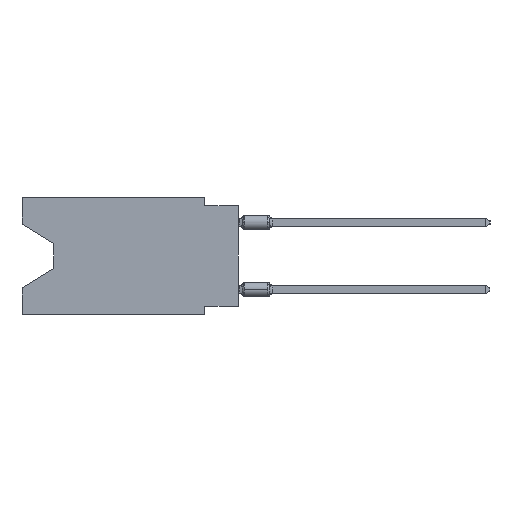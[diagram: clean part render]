
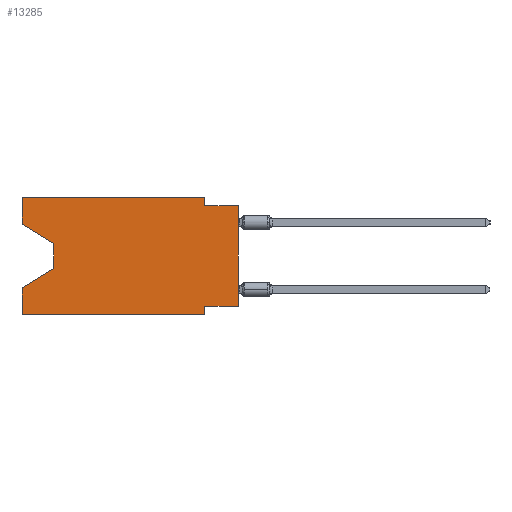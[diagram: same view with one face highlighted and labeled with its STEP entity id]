
A CAD part, left-side view. The second image highlights one B-rep face of the part: STEP entity #13285.
In plain terms, the highlighted planar face has unit normal (-1, 0, 0).
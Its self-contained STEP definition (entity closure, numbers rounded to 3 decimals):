
#343 = ORIENTED_EDGE ( 'NONE', *, *, #43292, .F. ) ;
#811 = CARTESIAN_POINT ( 'NONE',  ( 0., 16.383, 0. ) ) ;
#838 = LINE ( 'NONE', #42924, #15543 ) ;
#1033 = VERTEX_POINT ( 'NONE', #21829 ) ;
#1484 = EDGE_CURVE ( 'NONE', #16637, #2525, #44673, .T. ) ;
#1725 = LINE ( 'NONE', #29605, #27067 ) ;
#2525 = VERTEX_POINT ( 'NONE', #28909 ) ;
#2679 = CARTESIAN_POINT ( 'NONE',  ( 0., 16.383, -2.038 ) ) ;
#2691 = ORIENTED_EDGE ( 'NONE', *, *, #10028, .F. ) ;
#3459 = CARTESIAN_POINT ( 'NONE',  ( 0., 13.97, -5.385 ) ) ;
#3548 = EDGE_CURVE ( 'NONE', #30534, #17554, #838, .T. ) ;
#3558 = LINE ( 'NONE', #811, #14424 ) ;
#4808 = LINE ( 'NONE', #44132, #27550 ) ;
#5252 = CARTESIAN_POINT ( 'NONE',  ( 0., 2.54, -8.89 ) ) ;
#5733 = VECTOR ( 'NONE', #19193, 1000. ) ;
#7561 = DIRECTION ( 'NONE',  ( 0., 0., -1. ) ) ;
#7698 = ORIENTED_EDGE ( 'NONE', *, *, #27133, .F. ) ;
#7884 = CARTESIAN_POINT ( 'NONE',  ( 0., 0., -8.255 ) ) ;
#8462 = ORIENTED_EDGE ( 'NONE', *, *, #21504, .T. ) ;
#8587 = VERTEX_POINT ( 'NONE', #20730 ) ;
#9474 = DIRECTION ( 'NONE',  ( 0., -1., 0. ) ) ;
#9531 = CARTESIAN_POINT ( 'NONE',  ( 0., 2.54, -8.255 ) ) ;
#9591 = DIRECTION ( 'NONE',  ( 0., 0., 1. ) ) ;
#10028 = EDGE_CURVE ( 'NONE', #37496, #35633, #38396, .T. ) ;
#10310 = LINE ( 'NONE', #3459, #37599 ) ;
#10684 = ORIENTED_EDGE ( 'NONE', *, *, #33413, .T. ) ;
#11477 = CARTESIAN_POINT ( 'NONE',  ( 0., 13.97, -3.505 ) ) ;
#11752 = ORIENTED_EDGE ( 'NONE', *, *, #21544, .F. ) ;
#12558 = DIRECTION ( 'NONE',  ( 0., 0., 1. ) ) ;
#12906 = LINE ( 'NONE', #26847, #31722 ) ;
#13285 = ADVANCED_FACE ( 'NONE', ( #38209 ), #27908, .F. ) ;
#13310 = DIRECTION ( 'NONE',  ( 0., 0., -1. ) ) ;
#13400 = EDGE_CURVE ( 'NONE', #35983, #1033, #30785, .T. ) ;
#13512 = VECTOR ( 'NONE', #13310, 1000. ) ;
#13715 = EDGE_CURVE ( 'NONE', #35983, #8587, #1725, .T. ) ;
#13785 = VERTEX_POINT ( 'NONE', #16126 ) ;
#14193 = CARTESIAN_POINT ( 'NONE',  ( 0., 16.383, 0. ) ) ;
#14424 = VECTOR ( 'NONE', #21159, 1000. ) ;
#15543 = VECTOR ( 'NONE', #32831, 1000. ) ;
#15693 = VERTEX_POINT ( 'NONE', #9531 ) ;
#16126 = CARTESIAN_POINT ( 'NONE',  ( 0., 0., -8.255 ) ) ;
#16188 = VECTOR ( 'NONE', #39657, 1000. ) ;
#16637 = VERTEX_POINT ( 'NONE', #11477 ) ;
#17009 = ORIENTED_EDGE ( 'NONE', *, *, #3548, .F. ) ;
#17554 = VERTEX_POINT ( 'NONE', #37982 ) ;
#17857 = CARTESIAN_POINT ( 'NONE',  ( 0., 0., -0.635 ) ) ;
#19193 = DIRECTION ( 'NONE',  ( 0., 0., -1. ) ) ;
#19776 = CARTESIAN_POINT ( 'NONE',  ( 0., 16.383, 0. ) ) ;
#20458 = VERTEX_POINT ( 'NONE', #17857 ) ;
#20730 = CARTESIAN_POINT ( 'NONE',  ( 0., 2.54, -8.89 ) ) ;
#20774 = EDGE_LOOP ( 'NONE', ( #22227, #24663, #10684, #29657, #33717, #11752, #7698, #8462, #44574, #17009, #343, #2691 ) ) ;
#21159 = DIRECTION ( 'NONE',  ( 0., -1., 0. ) ) ;
#21504 = EDGE_CURVE ( 'NONE', #13785, #20458, #25608, .T. ) ;
#21544 = EDGE_CURVE ( 'NONE', #15693, #8587, #36564, .T. ) ;
#21829 = CARTESIAN_POINT ( 'NONE',  ( 0., 16.383, -6.852 ) ) ;
#22227 = ORIENTED_EDGE ( 'NONE', *, *, #43879, .T. ) ;
#24663 = ORIENTED_EDGE ( 'NONE', *, *, #1484, .T. ) ;
#25608 = LINE ( 'NONE', #43911, #44466 ) ;
#26198 = VECTOR ( 'NONE', #9591, 1000. ) ;
#26293 = AXIS2_PLACEMENT_3D ( 'NONE', #14193, #27689, #7561 ) ;
#26356 = CARTESIAN_POINT ( 'NONE',  ( 0., 16.383, -8.89 ) ) ;
#26721 = DIRECTION ( 'NONE',  ( 0., -0.855, -0.519 ) ) ;
#26847 = CARTESIAN_POINT ( 'NONE',  ( 0., 0., -0.635 ) ) ;
#26969 = CARTESIAN_POINT ( 'NONE',  ( 0., 16.383, 0. ) ) ;
#27067 = VECTOR ( 'NONE', #36921, 1000. ) ;
#27133 = EDGE_CURVE ( 'NONE', #13785, #15693, #36216, .T. ) ;
#27550 = VECTOR ( 'NONE', #26721, 1000. ) ;
#27689 = DIRECTION ( 'NONE',  ( 1., 0., 0. ) ) ;
#27789 = VECTOR ( 'NONE', #41088, 1000. ) ;
#27908 = PLANE ( 'NONE',  #26293 ) ;
#28909 = CARTESIAN_POINT ( 'NONE',  ( 0., 13.97, -5.385 ) ) ;
#29605 = CARTESIAN_POINT ( 'NONE',  ( 0., 16.383, -8.89 ) ) ;
#29657 = ORIENTED_EDGE ( 'NONE', *, *, #13400, .F. ) ;
#30534 = VERTEX_POINT ( 'NONE', #36833 ) ;
#30785 = LINE ( 'NONE', #44767, #27789 ) ;
#31722 = VECTOR ( 'NONE', #9474, 1000. ) ;
#32831 = DIRECTION ( 'NONE',  ( 0., 0., -1. ) ) ;
#32964 = EDGE_CURVE ( 'NONE', #17554, #20458, #12906, .T. ) ;
#33413 = EDGE_CURVE ( 'NONE', #2525, #1033, #10310, .T. ) ;
#33717 = ORIENTED_EDGE ( 'NONE', *, *, #13715, .T. ) ;
#33890 = CARTESIAN_POINT ( 'NONE',  ( 0., 13.97, -3.505 ) ) ;
#35633 = VERTEX_POINT ( 'NONE', #19776 ) ;
#35983 = VERTEX_POINT ( 'NONE', #26356 ) ;
#36216 = LINE ( 'NONE', #7884, #16188 ) ;
#36564 = LINE ( 'NONE', #5252, #5733 ) ;
#36833 = CARTESIAN_POINT ( 'NONE',  ( 0., 2.54, 0. ) ) ;
#36921 = DIRECTION ( 'NONE',  ( 0., -1., 0. ) ) ;
#37496 = VERTEX_POINT ( 'NONE', #2679 ) ;
#37599 = VECTOR ( 'NONE', #45110, 1000. ) ;
#37982 = CARTESIAN_POINT ( 'NONE',  ( 0., 2.54, -0.635 ) ) ;
#38209 = FACE_OUTER_BOUND ( 'NONE', #20774, .T. ) ;
#38396 = LINE ( 'NONE', #26969, #26198 ) ;
#39657 = DIRECTION ( 'NONE',  ( 0., 1., 0. ) ) ;
#41088 = DIRECTION ( 'NONE',  ( 0., 0., 1. ) ) ;
#42924 = CARTESIAN_POINT ( 'NONE',  ( 0., 2.54, 0. ) ) ;
#43292 = EDGE_CURVE ( 'NONE', #35633, #30534, #3558, .T. ) ;
#43879 = EDGE_CURVE ( 'NONE', #37496, #16637, #4808, .T. ) ;
#43911 = CARTESIAN_POINT ( 'NONE',  ( 0., 0., 0. ) ) ;
#44132 = CARTESIAN_POINT ( 'NONE',  ( 0., 16.383, -2.038 ) ) ;
#44466 = VECTOR ( 'NONE', #12558, 1000. ) ;
#44574 = ORIENTED_EDGE ( 'NONE', *, *, #32964, .F. ) ;
#44673 = LINE ( 'NONE', #33890, #13512 ) ;
#44767 = CARTESIAN_POINT ( 'NONE',  ( 0., 16.383, 0. ) ) ;
#45110 = DIRECTION ( 'NONE',  ( 0., 0.855, -0.519 ) ) ;
